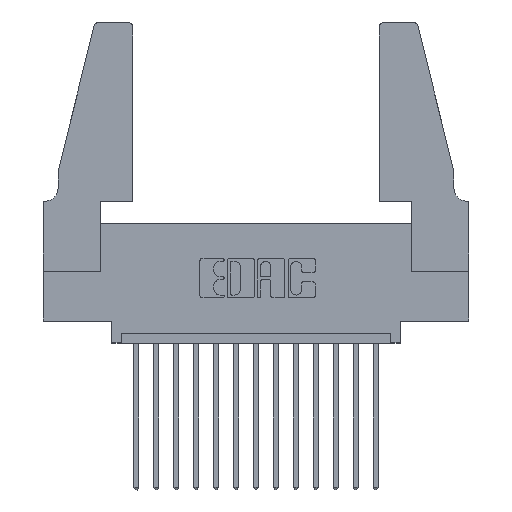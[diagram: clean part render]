
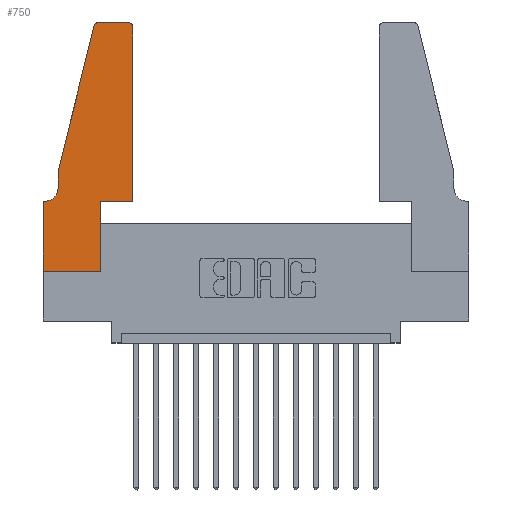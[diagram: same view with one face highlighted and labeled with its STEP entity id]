
A CAD part, top view. The second image highlights one B-rep face of the part: STEP entity #750.
In plain terms, the highlighted planar face has unit normal (0, 0, 1).
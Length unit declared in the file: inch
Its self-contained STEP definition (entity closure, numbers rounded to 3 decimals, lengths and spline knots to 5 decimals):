
#100 = ORIENTED_EDGE ( 'NONE', *, *, #7789, .T. ) ;
#332 = DIRECTION ( 'NONE',  ( -1., 0., 0. ) ) ;
#344 = ORIENTED_EDGE ( 'NONE', *, *, #8019, .T. ) ;
#386 = EDGE_CURVE ( 'NONE', #5417, #10737, #14293, .T. ) ;
#393 = DIRECTION ( 'NONE',  ( 1., 0., 0. ) ) ;
#404 = CARTESIAN_POINT ( 'NONE',  ( 0.0755, 0.42, 0.37 ) ) ;
#544 = DIRECTION ( 'NONE',  ( 1., 0., 0. ) ) ;
#750 = ADVANCED_FACE ( 'NONE', ( #9472 ), #3081, .T. ) ;
#1104 = CARTESIAN_POINT ( 'NONE',  ( 0.2865, 0.35, 0.37 ) ) ;
#1303 = EDGE_CURVE ( 'NONE', #5935, #4029, #7528, .T. ) ;
#1347 = CARTESIAN_POINT ( 'NONE',  ( 0.4205, 1.22, 0.37 ) ) ;
#1464 = CIRCLE ( 'NONE', #4376, 0.03 ) ;
#1643 = CARTESIAN_POINT ( 'NONE',  ( 0.0055, 0.42, 0.37 ) ) ;
#1651 = LINE ( 'NONE', #4104, #2994 ) ;
#1844 = DIRECTION ( 'NONE',  ( 1., 0., 0. ) ) ;
#1889 = CIRCLE ( 'NONE', #11762, 0.07 ) ;
#1923 = EDGE_CURVE ( 'NONE', #10737, #12766, #1889, .T. ) ;
#2462 = VERTEX_POINT ( 'NONE', #3833 ) ;
#2886 = VERTEX_POINT ( 'NONE', #7026 ) ;
#2994 = VECTOR ( 'NONE', #15057, 39.37008 ) ;
#3081 = PLANE ( 'NONE',  #8585 ) ;
#3703 = VERTEX_POINT ( 'NONE', #10650 ) ;
#3802 = EDGE_CURVE ( 'NONE', #2886, #2462, #9581, .T. ) ;
#3833 = CARTESIAN_POINT ( 'NONE',  ( 0.4505, 0.35, 0.37 ) ) ;
#4029 = VERTEX_POINT ( 'NONE', #14850 ) ;
#4051 = EDGE_CURVE ( 'NONE', #11927, #2886, #11488, .T. ) ;
#4104 = CARTESIAN_POINT ( 'NONE',  ( 0.4505, 0.35, 0.37 ) ) ;
#4174 = VECTOR ( 'NONE', #8266, 39.37008 ) ;
#4376 = AXIS2_PLACEMENT_3D ( 'NONE', #1347, #6215, #14862 ) ;
#4643 = EDGE_CURVE ( 'NONE', #2462, #4713, #1651, .T. ) ;
#4713 = VERTEX_POINT ( 'NONE', #8984 ) ;
#4917 = ORIENTED_EDGE ( 'NONE', *, *, #5640, .T. ) ;
#5072 = VECTOR ( 'NONE', #13748, 39.37008 ) ;
#5417 = VERTEX_POINT ( 'NONE', #11766 ) ;
#5491 = ORIENTED_EDGE ( 'NONE', *, *, #386, .T. ) ;
#5640 = EDGE_CURVE ( 'NONE', #6430, #14095, #6211, .T. ) ;
#5935 = VERTEX_POINT ( 'NONE', #11014 ) ;
#5998 = CARTESIAN_POINT ( 'NONE',  ( 0.0055, 0.35, 0.37 ) ) ;
#6198 = DIRECTION ( 'NONE',  ( 0., -1., 0. ) ) ;
#6211 = LINE ( 'NONE', #12148, #12599 ) ;
#6215 = DIRECTION ( 'NONE',  ( 0., 0., 1. ) ) ;
#6430 = VERTEX_POINT ( 'NONE', #15744 ) ;
#6587 = DIRECTION ( 'NONE',  ( 0., 0., -1. ) ) ;
#7026 = CARTESIAN_POINT ( 'NONE',  ( 0.2865, 0.35, 0.37 ) ) ;
#7528 = LINE ( 'NONE', #7937, #7901 ) ;
#7604 = EDGE_CURVE ( 'NONE', #4713, #5935, #1464, .T. ) ;
#7703 = ORIENTED_EDGE ( 'NONE', *, *, #4643, .T. ) ;
#7789 = EDGE_CURVE ( 'NONE', #3703, #5417, #13987, .T. ) ;
#7901 = VECTOR ( 'NONE', #14112, 39.37008 ) ;
#7937 = CARTESIAN_POINT ( 'NONE',  ( 0.2605, 1.25, 0.37 ) ) ;
#8019 = EDGE_CURVE ( 'NONE', #14095, #11927, #11084, .T. ) ;
#8151 = CARTESIAN_POINT ( 'NONE',  ( 0.2865, 0., 0.37 ) ) ;
#8266 = DIRECTION ( 'NONE',  ( -0.239, -0.971, 0. ) ) ;
#8585 = AXIS2_PLACEMENT_3D ( 'NONE', #11753, #11799, #544 ) ;
#8984 = CARTESIAN_POINT ( 'NONE',  ( 0.4505, 1.22, 0.37 ) ) ;
#9047 = EDGE_CURVE ( 'NONE', #12766, #6430, #12783, .T. ) ;
#9079 = CARTESIAN_POINT ( 'NONE',  ( 0.284, 1.22, 0.37 ) ) ;
#9248 = DIRECTION ( 'NONE',  ( 0., 0., 1. ) ) ;
#9334 = DIRECTION ( 'NONE',  ( 1., 0., 0. ) ) ;
#9472 = FACE_OUTER_BOUND ( 'NONE', #14562, .T. ) ;
#9581 = LINE ( 'NONE', #10427, #12475 ) ;
#10186 = ORIENTED_EDGE ( 'NONE', *, *, #4051, .T. ) ;
#10277 = VECTOR ( 'NONE', #6198, 39.37008 ) ;
#10427 = CARTESIAN_POINT ( 'NONE',  ( 0.4505, 0.35, 0.37 ) ) ;
#10445 = CARTESIAN_POINT ( 'NONE',  ( 0.0755, 0.35, 0.37 ) ) ;
#10591 = AXIS2_PLACEMENT_3D ( 'NONE', #9079, #9248, #393 ) ;
#10650 = CARTESIAN_POINT ( 'NONE',  ( 0.25487, 1.22718, 0.37 ) ) ;
#10737 = VERTEX_POINT ( 'NONE', #404 ) ;
#10837 = ORIENTED_EDGE ( 'NONE', *, *, #1303, .T. ) ;
#11014 = CARTESIAN_POINT ( 'NONE',  ( 0.4205, 1.25, 0.37 ) ) ;
#11084 = LINE ( 'NONE', #12041, #15521 ) ;
#11139 = CIRCLE ( 'NONE', #10591, 0.03 ) ;
#11177 = DIRECTION ( 'NONE',  ( 0., 1., 0. ) ) ;
#11488 = LINE ( 'NONE', #1104, #15354 ) ;
#11519 = CARTESIAN_POINT ( 'NONE',  ( 0., 0., 0.37 ) ) ;
#11531 = DIRECTION ( 'NONE',  ( 0., -1., 0. ) ) ;
#11753 = CARTESIAN_POINT ( 'NONE',  ( 0., 0.35, 0.37 ) ) ;
#11762 = AXIS2_PLACEMENT_3D ( 'NONE', #1643, #6587, #332 ) ;
#11766 = CARTESIAN_POINT ( 'NONE',  ( 0.0755, 0.5, 0.37 ) ) ;
#11799 = DIRECTION ( 'NONE',  ( 0., 0., 1. ) ) ;
#11927 = VERTEX_POINT ( 'NONE', #8151 ) ;
#12041 = CARTESIAN_POINT ( 'NONE',  ( 0., 0., 0.37 ) ) ;
#12077 = CARTESIAN_POINT ( 'NONE',  ( 0.0755, 0.5, 0.37 ) ) ;
#12148 = CARTESIAN_POINT ( 'NONE',  ( 0., 0., 0.37 ) ) ;
#12421 = EDGE_CURVE ( 'NONE', #4029, #3703, #11139, .T. ) ;
#12475 = VECTOR ( 'NONE', #1844, 39.37008 ) ;
#12599 = VECTOR ( 'NONE', #11531, 39.37008 ) ;
#12766 = VERTEX_POINT ( 'NONE', #5998 ) ;
#12783 = LINE ( 'NONE', #10445, #5072 ) ;
#13748 = DIRECTION ( 'NONE',  ( -1., 0., 0. ) ) ;
#13987 = LINE ( 'NONE', #12077, #4174 ) ;
#14095 = VERTEX_POINT ( 'NONE', #11519 ) ;
#14112 = DIRECTION ( 'NONE',  ( -1., 0., 0. ) ) ;
#14257 = ORIENTED_EDGE ( 'NONE', *, *, #7604, .T. ) ;
#14293 = LINE ( 'NONE', #15943, #10277 ) ;
#14368 = ORIENTED_EDGE ( 'NONE', *, *, #3802, .T. ) ;
#14562 = EDGE_LOOP ( 'NONE', ( #10837, #15160, #100, #5491, #15904, #15930, #4917, #344, #10186, #14368, #7703, #14257 ) ) ;
#14850 = CARTESIAN_POINT ( 'NONE',  ( 0.284, 1.25, 0.37 ) ) ;
#14862 = DIRECTION ( 'NONE',  ( 1., 0., 0. ) ) ;
#15057 = DIRECTION ( 'NONE',  ( 0., 1., 0. ) ) ;
#15160 = ORIENTED_EDGE ( 'NONE', *, *, #12421, .T. ) ;
#15354 = VECTOR ( 'NONE', #11177, 39.37008 ) ;
#15521 = VECTOR ( 'NONE', #9334, 39.37008 ) ;
#15744 = CARTESIAN_POINT ( 'NONE',  ( 0., 0.35, 0.37 ) ) ;
#15904 = ORIENTED_EDGE ( 'NONE', *, *, #1923, .T. ) ;
#15930 = ORIENTED_EDGE ( 'NONE', *, *, #9047, .T. ) ;
#15943 = CARTESIAN_POINT ( 'NONE',  ( 0.0755, 0.5, 0.37 ) ) ;
